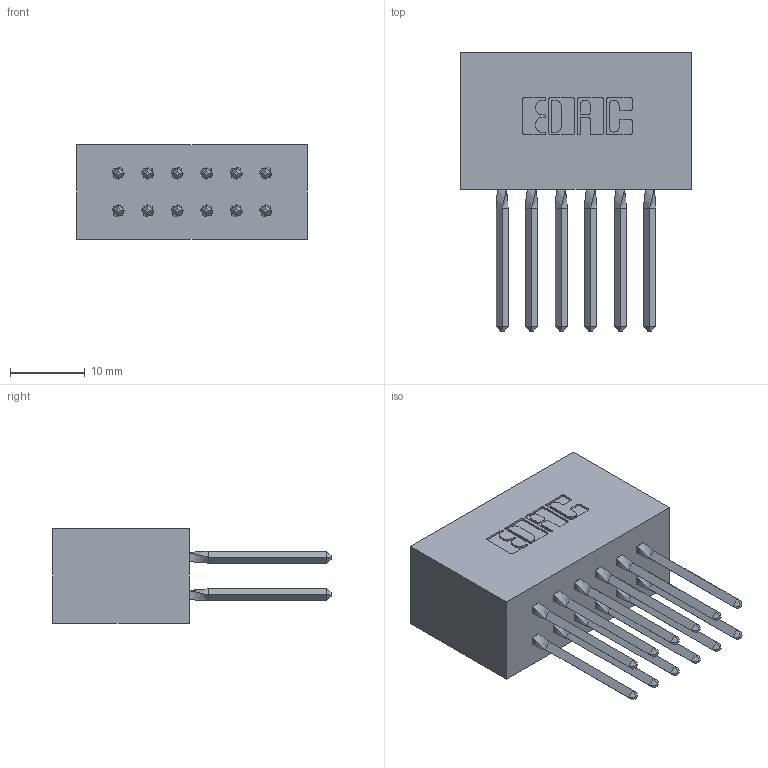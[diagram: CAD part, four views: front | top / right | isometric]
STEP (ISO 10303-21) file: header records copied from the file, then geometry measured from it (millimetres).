
FILE_DESCRIPTION (( 'STEP AP203' ), '1' );
FILE_NAME ('317-012-540-801.STEP', '2020-02-27T14:03:05', ( '' ), ( '' ), 'SwSTEP 2.0', 'SolidWorks 2016', '' );
FILE_SCHEMA (( 'CONFIG_CONTROL_DESIGN' ));
Length unit declared in the file: inch
Products named in the file (3): 317 Part_Lugless; 317-012-540-801; 317-290-001_540
Assembly tree (13 placements, depth 2):
  317-012-540-801
    317 Part_Lugless
    317-290-001_540  x12
Bounding box: 30.99 x 37.34 x 12.7 mm (x, y, z)
Volume: 5777.1 mm3; surface area: 7510 mm2
Topology: 13 solids, 13 shells, 1158 faces, 3203 edges, 2066 vertices
Faces by surface type: plane 926, cylinder 184, bspline 48
Entity records: 13286 total; most frequent: CARTESIAN_POINT 2727, ORIENTED_EDGE 2226, DIRECTION 1855, EDGE_CURVE 1113, LINE 865, VECTOR 865, VERTEX_POINT 735, AXIS2_PLACEMENT_3D 495
